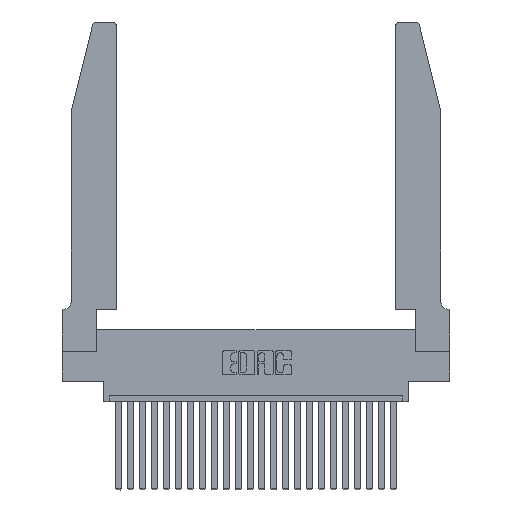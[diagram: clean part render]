
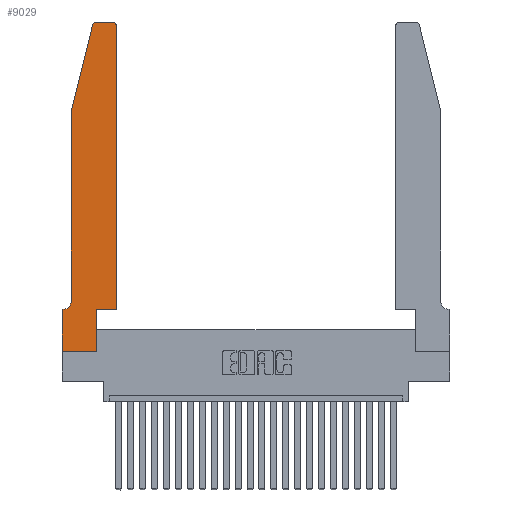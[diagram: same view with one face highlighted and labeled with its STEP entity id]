
A CAD part, top view. The second image highlights one B-rep face of the part: STEP entity #9029.
In plain terms, the highlighted planar face has unit normal (0, 0, 1).
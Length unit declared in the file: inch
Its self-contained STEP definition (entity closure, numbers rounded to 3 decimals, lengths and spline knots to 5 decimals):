
#95 = VERTEX_POINT ( 'NONE', #14227 ) ;
#189 = CARTESIAN_POINT ( 'NONE',  ( 0.2865, 0., 0.37 ) ) ;
#406 = CARTESIAN_POINT ( 'NONE',  ( 0., 0.35, 0.37 ) ) ;
#551 = ORIENTED_EDGE ( 'NONE', *, *, #21721, .T. ) ;
#611 = CARTESIAN_POINT ( 'NONE',  ( 0.0755, 2., 0.37 ) ) ;
#721 = LINE ( 'NONE', #21756, #19971 ) ;
#825 = EDGE_CURVE ( 'NONE', #6559, #12379, #15941, .T. ) ;
#1170 = VERTEX_POINT ( 'NONE', #23165 ) ;
#1413 = CARTESIAN_POINT ( 'NONE',  ( 0.2605, 2.75, 0.37 ) ) ;
#1438 = CARTESIAN_POINT ( 'NONE',  ( 0.0755, 0.42, 0.37 ) ) ;
#1946 = VERTEX_POINT ( 'NONE', #1438 ) ;
#2468 = DIRECTION ( 'NONE',  ( 0., 0., 1. ) ) ;
#3142 = EDGE_LOOP ( 'NONE', ( #4569, #18053, #14172, #551, #15308, #8813, #17075, #4096, #22710, #18420, #14510, #18586 ) ) ;
#3249 = LINE ( 'NONE', #12366, #21526 ) ;
#4096 = ORIENTED_EDGE ( 'NONE', *, *, #6884, .T. ) ;
#4095 = AXIS2_PLACEMENT_3D ( 'NONE', #16054, #10242, #14180 ) ;
#4151 = EDGE_CURVE ( 'NONE', #6666, #7163, #21557, .T. ) ;
#4569 = ORIENTED_EDGE ( 'NONE', *, *, #4151, .T. ) ;
#4575 = VECTOR ( 'NONE', #19893, 39.37008 ) ;
#5273 = VECTOR ( 'NONE', #12663, 39.37008 ) ;
#5597 = AXIS2_PLACEMENT_3D ( 'NONE', #406, #6250, #8226 ) ;
#6250 = DIRECTION ( 'NONE',  ( 0., 0., 1. ) ) ;
#6559 = VERTEX_POINT ( 'NONE', #21294 ) ;
#6666 = VERTEX_POINT ( 'NONE', #17848 ) ;
#6833 = DIRECTION ( 'NONE',  ( 0., 1., 0. ) ) ;
#6884 = EDGE_CURVE ( 'NONE', #23509, #14406, #20137, .T. ) ;
#7163 = VERTEX_POINT ( 'NONE', #20104 ) ;
#8185 = VECTOR ( 'NONE', #22520, 39.37008 ) ;
#8226 = DIRECTION ( 'NONE',  ( 1., 0., 0. ) ) ;
#8253 = CARTESIAN_POINT ( 'NONE',  ( 0., 0., 0.37 ) ) ;
#8258 = VERTEX_POINT ( 'NONE', #12271 ) ;
#8343 = LINE ( 'NONE', #12752, #5273 ) ;
#8813 = ORIENTED_EDGE ( 'NONE', *, *, #11583, .T. ) ;
#9029 = ADVANCED_FACE ( 'NONE', ( #10274 ), #10016, .T. ) ;
#9217 = DIRECTION ( 'NONE',  ( 0., 1., 0. ) ) ;
#9782 = EDGE_CURVE ( 'NONE', #14406, #1170, #721, .T. ) ;
#10016 = PLANE ( 'NONE',  #5597 ) ;
#10026 = EDGE_CURVE ( 'NONE', #12379, #6666, #16328, .T. ) ;
#10242 = DIRECTION ( 'NONE',  ( 0., 0., 1. ) ) ;
#10274 = FACE_OUTER_BOUND ( 'NONE', #3142, .T. ) ;
#10575 = DIRECTION ( 'NONE',  ( -0.239, -0.971, 0. ) ) ;
#11110 = LINE ( 'NONE', #23445, #20843 ) ;
#11207 = EDGE_CURVE ( 'NONE', #1170, #6559, #8343, .T. ) ;
#11583 = EDGE_CURVE ( 'NONE', #95, #24755, #11110, .T. ) ;
#12195 = CARTESIAN_POINT ( 'NONE',  ( 0.0055, 0.42, 0.37 ) ) ;
#12271 = CARTESIAN_POINT ( 'NONE',  ( 0.25487, 2.72718, 0.37 ) ) ;
#12366 = CARTESIAN_POINT ( 'NONE',  ( 0.0755, 2., 0.37 ) ) ;
#12379 = VERTEX_POINT ( 'NONE', #17750 ) ;
#12383 = CARTESIAN_POINT ( 'NONE',  ( 0.284, 2.72, 0.37 ) ) ;
#12663 = DIRECTION ( 'NONE',  ( 1., 0., 0. ) ) ;
#12752 = CARTESIAN_POINT ( 'NONE',  ( 0.4505, 0.35, 0.37 ) ) ;
#12799 = CARTESIAN_POINT ( 'NONE',  ( 0., 0., 0.37 ) ) ;
#13200 = EDGE_CURVE ( 'NONE', #7163, #8258, #19634, .T. ) ;
#13862 = VECTOR ( 'NONE', #10575, 39.37008 ) ;
#14011 = DIRECTION ( 'NONE',  ( -1., 0., 0. ) ) ;
#14172 = ORIENTED_EDGE ( 'NONE', *, *, #23897, .T. ) ;
#14180 = DIRECTION ( 'NONE',  ( 1., 0., 0. ) ) ;
#14188 = DIRECTION ( 'NONE',  ( 0., 0., -1. ) ) ;
#14227 = CARTESIAN_POINT ( 'NONE',  ( 0.0055, 0.35, 0.37 ) ) ;
#14406 = VERTEX_POINT ( 'NONE', #189 ) ;
#14459 = EDGE_CURVE ( 'NONE', #24755, #23509, #21086, .T. ) ;
#14460 = VERTEX_POINT ( 'NONE', #18018 ) ;
#14510 = ORIENTED_EDGE ( 'NONE', *, *, #825, .T. ) ;
#15222 = CARTESIAN_POINT ( 'NONE',  ( 0., 0.35, 0.37 ) ) ;
#15308 = ORIENTED_EDGE ( 'NONE', *, *, #21029, .T. ) ;
#15735 = DIRECTION ( 'NONE',  ( -1., 0., 0. ) ) ;
#15941 = LINE ( 'NONE', #20815, #17746 ) ;
#16054 = CARTESIAN_POINT ( 'NONE',  ( 0.4205, 2.72, 0.37 ) ) ;
#16208 = DIRECTION ( 'NONE',  ( 0., -1., 0. ) ) ;
#16301 = AXIS2_PLACEMENT_3D ( 'NONE', #12195, #14188, #14011 ) ;
#16328 = CIRCLE ( 'NONE', #4095, 0.03 ) ;
#17075 = ORIENTED_EDGE ( 'NONE', *, *, #14459, .T. ) ;
#17746 = VECTOR ( 'NONE', #9217, 39.37008 ) ;
#17750 = CARTESIAN_POINT ( 'NONE',  ( 0.4505, 2.72, 0.37 ) ) ;
#17848 = CARTESIAN_POINT ( 'NONE',  ( 0.4205, 2.75, 0.37 ) ) ;
#18018 = CARTESIAN_POINT ( 'NONE',  ( 0.0755, 2., 0.37 ) ) ;
#18053 = ORIENTED_EDGE ( 'NONE', *, *, #13200, .T. ) ;
#18420 = ORIENTED_EDGE ( 'NONE', *, *, #11207, .T. ) ;
#18586 = ORIENTED_EDGE ( 'NONE', *, *, #10026, .T. ) ;
#19451 = CIRCLE ( 'NONE', #16301, 0.07 ) ;
#19634 = CIRCLE ( 'NONE', #24015, 0.03 ) ;
#19642 = LINE ( 'NONE', #611, #13862 ) ;
#19659 = CARTESIAN_POINT ( 'NONE',  ( 0., 0., 0.37 ) ) ;
#19893 = DIRECTION ( 'NONE',  ( 0., -1., 0. ) ) ;
#19971 = VECTOR ( 'NONE', #6833, 39.37008 ) ;
#20045 = DIRECTION ( 'NONE',  ( 1., 0., 0. ) ) ;
#20104 = CARTESIAN_POINT ( 'NONE',  ( 0.284, 2.75, 0.37 ) ) ;
#20137 = LINE ( 'NONE', #8253, #20438 ) ;
#20438 = VECTOR ( 'NONE', #23462, 39.37008 ) ;
#20815 = CARTESIAN_POINT ( 'NONE',  ( 0.4505, 0.35, 0.37 ) ) ;
#20843 = VECTOR ( 'NONE', #15735, 39.37008 ) ;
#21029 = EDGE_CURVE ( 'NONE', #1946, #95, #19451, .T. ) ;
#21086 = LINE ( 'NONE', #19659, #4575 ) ;
#21294 = CARTESIAN_POINT ( 'NONE',  ( 0.4505, 0.35, 0.37 ) ) ;
#21526 = VECTOR ( 'NONE', #16208, 39.37008 ) ;
#21557 = LINE ( 'NONE', #1413, #8185 ) ;
#21721 = EDGE_CURVE ( 'NONE', #14460, #1946, #3249, .T. ) ;
#21756 = CARTESIAN_POINT ( 'NONE',  ( 0.2865, 0.35, 0.37 ) ) ;
#22520 = DIRECTION ( 'NONE',  ( -1., 0., 0. ) ) ;
#22710 = ORIENTED_EDGE ( 'NONE', *, *, #9782, .T. ) ;
#23165 = CARTESIAN_POINT ( 'NONE',  ( 0.2865, 0.35, 0.37 ) ) ;
#23445 = CARTESIAN_POINT ( 'NONE',  ( 0.0755, 0.35, 0.37 ) ) ;
#23462 = DIRECTION ( 'NONE',  ( 1., 0., 0. ) ) ;
#23509 = VERTEX_POINT ( 'NONE', #12799 ) ;
#23897 = EDGE_CURVE ( 'NONE', #8258, #14460, #19642, .T. ) ;
#24015 = AXIS2_PLACEMENT_3D ( 'NONE', #12383, #2468, #20045 ) ;
#24755 = VERTEX_POINT ( 'NONE', #15222 ) ;
